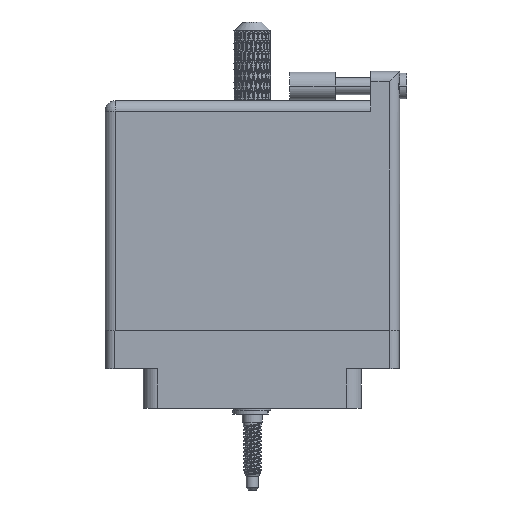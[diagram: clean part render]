
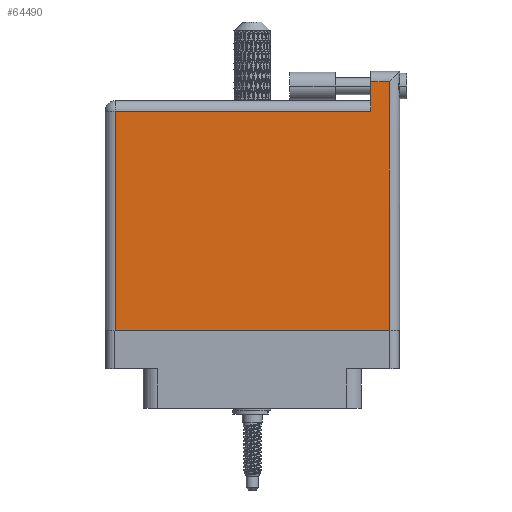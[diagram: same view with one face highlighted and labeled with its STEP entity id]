
A CAD part, front view. The second image highlights one B-rep face of the part: STEP entity #64490.
In plain terms, the highlighted face is planar.
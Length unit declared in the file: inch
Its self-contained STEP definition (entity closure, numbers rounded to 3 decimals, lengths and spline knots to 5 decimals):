
#2672 = VERTEX_POINT ( 'NONE', #45784 ) ;
#9340 = VECTOR ( 'NONE', #95672, 39.37008 ) ;
#10618 = DIRECTION ( 'NONE',  ( 1., 0., 0. ) ) ;
#12210 = EDGE_CURVE ( 'NONE', #32924, #86138, #73572, .T. ) ;
#15407 = VERTEX_POINT ( 'NONE', #50017 ) ;
#15484 = CARTESIAN_POINT ( 'NONE',  ( 1.811, 1.696, 0. ) ) ;
#16888 = VECTOR ( 'NONE', #10618, 39.37008 ) ;
#21154 = DIRECTION ( 'NONE',  ( -1., 0., 0. ) ) ;
#22456 = VECTOR ( 'NONE', #21154, 39.37008 ) ;
#22697 = VERTEX_POINT ( 'NONE', #27578 ) ;
#23750 = CARTESIAN_POINT ( 'NONE',  ( 1.938, 1.766, 0. ) ) ;
#25571 = PLANE ( 'NONE',  #77423 ) ;
#27360 = VERTEX_POINT ( 'NONE', #94850 ) ;
#27426 = DIRECTION ( 'NONE',  ( 0., -1., 0. ) ) ;
#27578 = CARTESIAN_POINT ( 'NONE',  ( 0.07, 0., 0. ) ) ;
#29783 = DIRECTION ( 'NONE',  ( 0., -1., 0. ) ) ;
#29883 = VECTOR ( 'NONE', #104212, 39.37008 ) ;
#30724 = LINE ( 'NONE', #23750, #9340 ) ;
#32924 = VERTEX_POINT ( 'NONE', #15484 ) ;
#34561 = CARTESIAN_POINT ( 'NONE',  ( 0., 0., 0. ) ) ;
#34986 = DIRECTION ( 'NONE',  ( 0., 0., -1. ) ) ;
#35387 = CARTESIAN_POINT ( 'NONE',  ( 1.811, 1.766, 0. ) ) ;
#41233 = LINE ( 'NONE', #72407, #29883 ) ;
#44189 = ORIENTED_EDGE ( 'NONE', *, *, #12210, .T. ) ;
#44766 = CARTESIAN_POINT ( 'NONE',  ( 0., 1.696, 0. ) ) ;
#45784 = CARTESIAN_POINT ( 'NONE',  ( 0.07, 1.496, 0. ) ) ;
#45889 = EDGE_CURVE ( 'NONE', #22697, #27360, #83643, .T. ) ;
#46609 = ORIENTED_EDGE ( 'NONE', *, *, #86993, .T. ) ;
#50017 = CARTESIAN_POINT ( 'NONE',  ( 1.938, 1.696, 0. ) ) ;
#50332 = ORIENTED_EDGE ( 'NONE', *, *, #51372, .T. ) ;
#51372 = EDGE_CURVE ( 'NONE', #15407, #32924, #56362, .T. ) ;
#54590 = ORIENTED_EDGE ( 'NONE', *, *, #59964, .T. ) ;
#56362 = LINE ( 'NONE', #44766, #22456 ) ;
#59964 = EDGE_CURVE ( 'NONE', #2672, #22697, #72106, .T. ) ;
#60399 = EDGE_LOOP ( 'NONE', ( #100307, #94880, #50332, #44189, #46609, #54590 ) ) ;
#60409 = CARTESIAN_POINT ( 'NONE',  ( 0.07, 0., 0. ) ) ;
#64490 = ADVANCED_FACE ( 'NONE', ( #82797 ), #25571, .F. ) ;
#64727 = VECTOR ( 'NONE', #29783, 39.37008 ) ;
#72106 = LINE ( 'NONE', #60409, #91085 ) ;
#72407 = CARTESIAN_POINT ( 'NONE',  ( 0., 1.496, 0. ) ) ;
#73572 = LINE ( 'NONE', #35387, #64727 ) ;
#77423 = AXIS2_PLACEMENT_3D ( 'NONE', #90728, #34986, #98195 ) ;
#80169 = EDGE_CURVE ( 'NONE', #27360, #15407, #30724, .T. ) ;
#82797 = FACE_OUTER_BOUND ( 'NONE', #60399, .T. ) ;
#83643 = LINE ( 'NONE', #34561, #16888 ) ;
#86138 = VERTEX_POINT ( 'NONE', #98562 ) ;
#86993 = EDGE_CURVE ( 'NONE', #86138, #2672, #41233, .T. ) ;
#90728 = CARTESIAN_POINT ( 'NONE',  ( 0., 1.566, 0. ) ) ;
#91085 = VECTOR ( 'NONE', #27426, 39.37008 ) ;
#94850 = CARTESIAN_POINT ( 'NONE',  ( 1.938, 0., 0. ) ) ;
#94880 = ORIENTED_EDGE ( 'NONE', *, *, #80169, .T. ) ;
#95672 = DIRECTION ( 'NONE',  ( 0., 1., 0. ) ) ;
#98195 = DIRECTION ( 'NONE',  ( -1., 0., 0. ) ) ;
#98562 = CARTESIAN_POINT ( 'NONE',  ( 1.811, 1.496, 0. ) ) ;
#100307 = ORIENTED_EDGE ( 'NONE', *, *, #45889, .T. ) ;
#104212 = DIRECTION ( 'NONE',  ( -1., 0., 0. ) ) ;
